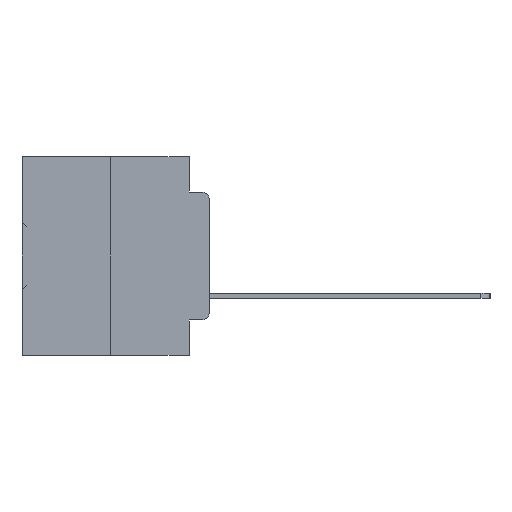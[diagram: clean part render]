
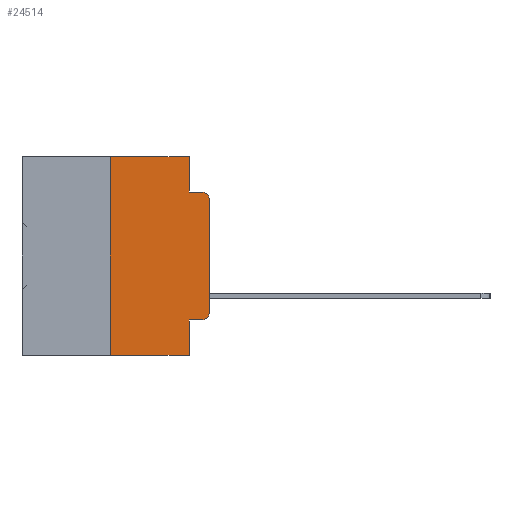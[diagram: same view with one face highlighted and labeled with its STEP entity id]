
A CAD part, left-side view. The second image highlights one B-rep face of the part: STEP entity #24514.
In plain terms, the highlighted planar face has unit normal (-1, 0, 0).
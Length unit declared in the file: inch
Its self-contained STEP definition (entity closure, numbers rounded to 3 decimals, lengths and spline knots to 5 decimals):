
#366 = VERTEX_POINT ( 'NONE', #16390 ) ;
#370 = CARTESIAN_POINT ( 'NONE',  ( 0., 0.051, -0.4115 ) ) ;
#830 = CARTESIAN_POINT ( 'NONE',  ( 0., 0.473, 0. ) ) ;
#1171 = AXIS2_PLACEMENT_3D ( 'NONE', #830, #6908, #27794 ) ;
#2037 = VERTEX_POINT ( 'NONE', #29651 ) ;
#2660 = ORIENTED_EDGE ( 'NONE', *, *, #25933, .T. ) ;
#3463 = AXIS2_PLACEMENT_3D ( 'NONE', #23189, #5281, #26146 ) ;
#3970 = CARTESIAN_POINT ( 'NONE',  ( 0., 0.473, 0. ) ) ;
#4083 = ORIENTED_EDGE ( 'NONE', *, *, #15937, .F. ) ;
#4591 = DIRECTION ( 'NONE',  ( -1., 0., 0. ) ) ;
#4766 = CARTESIAN_POINT ( 'NONE',  ( 0., 0.25, 0. ) ) ;
#4883 = CARTESIAN_POINT ( 'NONE',  ( 0., 0., -0.3915 ) ) ;
#5281 = DIRECTION ( 'NONE',  ( -1., 0., 0. ) ) ;
#5435 = ORIENTED_EDGE ( 'NONE', *, *, #17936, .F. ) ;
#5914 = EDGE_CURVE ( 'NONE', #11341, #30695, #9616, .T. ) ;
#6908 = DIRECTION ( 'NONE',  ( 1., 0., 0. ) ) ;
#7046 = VERTEX_POINT ( 'NONE', #12839 ) ;
#7187 = VECTOR ( 'NONE', #17413, 39.37008 ) ;
#7891 = EDGE_CURVE ( 'NONE', #35909, #11341, #37323, .T. ) ;
#8665 = FACE_OUTER_BOUND ( 'NONE', #30837, .T. ) ;
#9616 = CIRCLE ( 'NONE', #17892, 0.02 ) ;
#11341 = VERTEX_POINT ( 'NONE', #24753 ) ;
#11462 = DIRECTION ( 'NONE',  ( 0., -1., 0. ) ) ;
#11573 = VECTOR ( 'NONE', #11462, 39.37008 ) ;
#11886 = CARTESIAN_POINT ( 'NONE',  ( 0., 0.051, -0.5 ) ) ;
#11927 = EDGE_CURVE ( 'NONE', #35909, #12272, #38162, .T. ) ;
#12272 = VERTEX_POINT ( 'NONE', #11886 ) ;
#12556 = VECTOR ( 'NONE', #30897, 39.37008 ) ;
#12839 = CARTESIAN_POINT ( 'NONE',  ( 0., 0.25, 0. ) ) ;
#13091 = LINE ( 'NONE', #3970, #30784 ) ;
#14475 = CARTESIAN_POINT ( 'NONE',  ( 0., 0.051, -0.0885 ) ) ;
#14799 = ORIENTED_EDGE ( 'NONE', *, *, #11927, .F. ) ;
#14809 = LINE ( 'NONE', #4766, #21882 ) ;
#15074 = VERTEX_POINT ( 'NONE', #14475 ) ;
#15145 = LINE ( 'NONE', #32187, #7187 ) ;
#15937 = EDGE_CURVE ( 'NONE', #366, #7046, #14809, .T. ) ;
#16390 = CARTESIAN_POINT ( 'NONE',  ( 0., 0.25, -0.5 ) ) ;
#17413 = DIRECTION ( 'NONE',  ( 0., 0., -1. ) ) ;
#17892 = AXIS2_PLACEMENT_3D ( 'NONE', #22506, #4591, #25450 ) ;
#17936 = EDGE_CURVE ( 'NONE', #18615, #15074, #15145, .T. ) ;
#18615 = VERTEX_POINT ( 'NONE', #20673 ) ;
#19120 = CARTESIAN_POINT ( 'NONE',  ( 0., 0., 0. ) ) ;
#19127 = CARTESIAN_POINT ( 'NONE',  ( 0., 0.051, 0. ) ) ;
#19256 = DIRECTION ( 'NONE',  ( 0., 0., -1. ) ) ;
#19520 = ORIENTED_EDGE ( 'NONE', *, *, #7891, .T. ) ;
#19974 = EDGE_CURVE ( 'NONE', #15074, #23202, #22518, .T. ) ;
#20258 = EDGE_CURVE ( 'NONE', #7046, #18615, #13091, .T. ) ;
#20673 = CARTESIAN_POINT ( 'NONE',  ( 0., 0.051, 0. ) ) ;
#21747 = VECTOR ( 'NONE', #30992, 39.37008 ) ;
#21882 = VECTOR ( 'NONE', #22686, 39.37008 ) ;
#22504 = EDGE_CURVE ( 'NONE', #366, #12272, #36144, .T. ) ;
#22506 = CARTESIAN_POINT ( 'NONE',  ( 0., 0.02, -0.3915 ) ) ;
#22518 = LINE ( 'NONE', #26646, #37164 ) ;
#22686 = DIRECTION ( 'NONE',  ( 0., 0., 1. ) ) ;
#23189 = CARTESIAN_POINT ( 'NONE',  ( 0., 0.02, -0.1085 ) ) ;
#23202 = VERTEX_POINT ( 'NONE', #32569 ) ;
#24514 = ADVANCED_FACE ( 'NONE', ( #8665 ), #30627, .F. ) ;
#24753 = CARTESIAN_POINT ( 'NONE',  ( 0., 0.02, -0.4115 ) ) ;
#25061 = ORIENTED_EDGE ( 'NONE', *, *, #20258, .F. ) ;
#25450 = DIRECTION ( 'NONE',  ( 0., 0., -1. ) ) ;
#25933 = EDGE_CURVE ( 'NONE', #2037, #23202, #37707, .T. ) ;
#26146 = DIRECTION ( 'NONE',  ( 0., 0., -1. ) ) ;
#26646 = CARTESIAN_POINT ( 'NONE',  ( 0., 0.051, -0.0885 ) ) ;
#27794 = DIRECTION ( 'NONE',  ( 0., 0., -1. ) ) ;
#27929 = EDGE_CURVE ( 'NONE', #30695, #2037, #35283, .T. ) ;
#28035 = CARTESIAN_POINT ( 'NONE',  ( 0., 0.051, -0.4115 ) ) ;
#28309 = ORIENTED_EDGE ( 'NONE', *, *, #19974, .F. ) ;
#29631 = DIRECTION ( 'NONE',  ( 0., -1., 0. ) ) ;
#29651 = CARTESIAN_POINT ( 'NONE',  ( 0., 0., -0.1085 ) ) ;
#29703 = ORIENTED_EDGE ( 'NONE', *, *, #22504, .T. ) ;
#30627 = PLANE ( 'NONE',  #1171 ) ;
#30695 = VERTEX_POINT ( 'NONE', #4883 ) ;
#30784 = VECTOR ( 'NONE', #33701, 39.37008 ) ;
#30837 = EDGE_LOOP ( 'NONE', ( #38300, #2660, #28309, #5435, #25061, #4083, #29703, #14799, #19520, #37012 ) ) ;
#30897 = DIRECTION ( 'NONE',  ( 0., 0., 1. ) ) ;
#30992 = DIRECTION ( 'NONE',  ( 0., -1., 0. ) ) ;
#32187 = CARTESIAN_POINT ( 'NONE',  ( 0., 0.051, 0. ) ) ;
#32248 = CARTESIAN_POINT ( 'NONE',  ( 0., 0.473, -0.5 ) ) ;
#32569 = CARTESIAN_POINT ( 'NONE',  ( 0., 0.02, -0.0885 ) ) ;
#33701 = DIRECTION ( 'NONE',  ( 0., -1., 0. ) ) ;
#35283 = LINE ( 'NONE', #19120, #12556 ) ;
#35909 = VERTEX_POINT ( 'NONE', #370 ) ;
#36144 = LINE ( 'NONE', #32248, #11573 ) ;
#36368 = VECTOR ( 'NONE', #19256, 39.37008 ) ;
#37012 = ORIENTED_EDGE ( 'NONE', *, *, #5914, .T. ) ;
#37164 = VECTOR ( 'NONE', #29631, 39.37008 ) ;
#37323 = LINE ( 'NONE', #28035, #21747 ) ;
#37707 = CIRCLE ( 'NONE', #3463, 0.02 ) ;
#38162 = LINE ( 'NONE', #19127, #36368 ) ;
#38300 = ORIENTED_EDGE ( 'NONE', *, *, #27929, .T. ) ;
